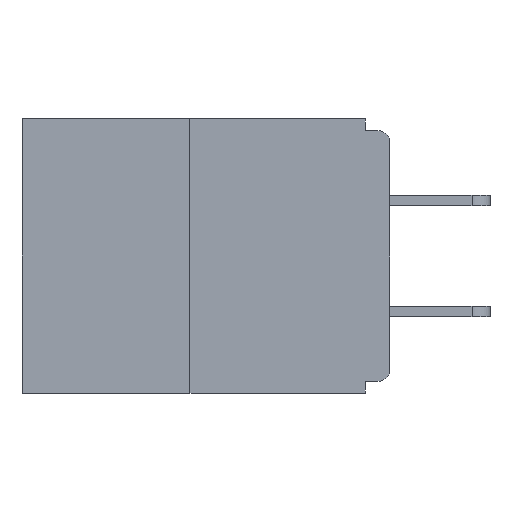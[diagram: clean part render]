
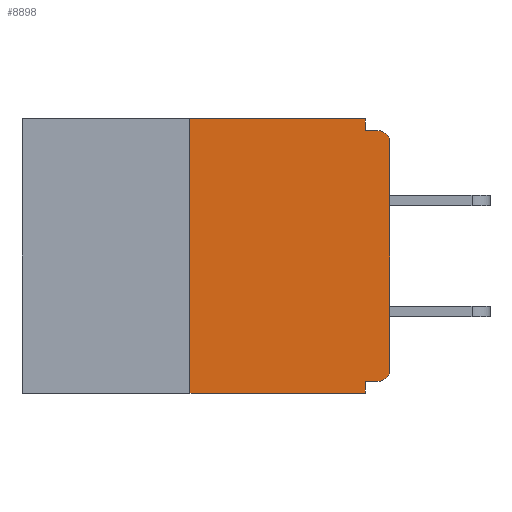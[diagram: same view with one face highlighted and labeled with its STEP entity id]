
A CAD part, left-side view. The second image highlights one B-rep face of the part: STEP entity #8898.
In plain terms, the highlighted planar face has unit normal (-1, 0, 0).
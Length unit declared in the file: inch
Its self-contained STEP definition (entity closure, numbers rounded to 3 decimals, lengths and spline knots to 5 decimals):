
#138 = AXIS2_PLACEMENT_3D ( 'NONE', #9693, #10923, #15683 ) ;
#494 = ORIENTED_EDGE ( 'NONE', *, *, #13513, .T. ) ;
#557 = VERTEX_POINT ( 'NONE', #8828 ) ;
#639 = CARTESIAN_POINT ( 'NONE',  ( 0., 0.46, 0. ) ) ;
#758 = CARTESIAN_POINT ( 'NONE',  ( 0., 0., -0.03 ) ) ;
#788 = VECTOR ( 'NONE', #9981, 39.37008 ) ;
#994 = CARTESIAN_POINT ( 'NONE',  ( 0., 0.25, 0. ) ) ;
#1169 = CARTESIAN_POINT ( 'NONE',  ( 0., 0.015, -0.328 ) ) ;
#1324 = CARTESIAN_POINT ( 'NONE',  ( 0., 0.031, 0. ) ) ;
#1523 = DIRECTION ( 'NONE',  ( 0., -1., 0. ) ) ;
#1751 = VERTEX_POINT ( 'NONE', #758 ) ;
#2694 = LINE ( 'NONE', #13413, #4240 ) ;
#2738 = VERTEX_POINT ( 'NONE', #1169 ) ;
#2758 = EDGE_CURVE ( 'NONE', #14366, #15210, #14642, .T. ) ;
#2929 = DIRECTION ( 'NONE',  ( -1., 0., 0. ) ) ;
#3044 = CARTESIAN_POINT ( 'NONE',  ( 0., 0.25, 0. ) ) ;
#3062 = PLANE ( 'NONE',  #13692 ) ;
#3267 = ORIENTED_EDGE ( 'NONE', *, *, #8157, .F. ) ;
#3478 = DIRECTION ( 'NONE',  ( 0., 0., 1. ) ) ;
#3661 = EDGE_CURVE ( 'NONE', #4261, #11013, #11527, .T. ) ;
#3828 = VERTEX_POINT ( 'NONE', #14357 ) ;
#3891 = ORIENTED_EDGE ( 'NONE', *, *, #13217, .F. ) ;
#4125 = CARTESIAN_POINT ( 'NONE',  ( 0., 0.015, -0.03 ) ) ;
#4240 = VECTOR ( 'NONE', #4927, 39.37008 ) ;
#4261 = VERTEX_POINT ( 'NONE', #12581 ) ;
#4388 = EDGE_CURVE ( 'NONE', #5724, #1751, #14214, .T. ) ;
#4489 = CARTESIAN_POINT ( 'NONE',  ( 0., 0.015, -0.015 ) ) ;
#4735 = FACE_OUTER_BOUND ( 'NONE', #6961, .T. ) ;
#4804 = CIRCLE ( 'NONE', #138, 0.015 ) ;
#4927 = DIRECTION ( 'NONE',  ( 0., 0., -1. ) ) ;
#5104 = ORIENTED_EDGE ( 'NONE', *, *, #3661, .F. ) ;
#5170 = DIRECTION ( 'NONE',  ( 0., -1., 0. ) ) ;
#5554 = ORIENTED_EDGE ( 'NONE', *, *, #11014, .F. ) ;
#5724 = VERTEX_POINT ( 'NONE', #14810 ) ;
#6026 = CARTESIAN_POINT ( 'NONE',  ( 0., 0., -0.015 ) ) ;
#6124 = ORIENTED_EDGE ( 'NONE', *, *, #11642, .F. ) ;
#6230 = ORIENTED_EDGE ( 'NONE', *, *, #12627, .T. ) ;
#6364 = LINE ( 'NONE', #15581, #13522 ) ;
#6420 = ORIENTED_EDGE ( 'NONE', *, *, #4388, .T. ) ;
#6907 = DIRECTION ( 'NONE',  ( 0., 0., -1. ) ) ;
#6934 = LINE ( 'NONE', #1324, #788 ) ;
#6961 = EDGE_LOOP ( 'NONE', ( #3267, #5104, #12795, #3891, #5554, #6230, #6420, #494, #7894, #6124 ) ) ;
#7649 = VECTOR ( 'NONE', #3478, 39.37008 ) ;
#7894 = ORIENTED_EDGE ( 'NONE', *, *, #2758, .F. ) ;
#7984 = CARTESIAN_POINT ( 'NONE',  ( 0., 0., -0.328 ) ) ;
#8157 = EDGE_CURVE ( 'NONE', #11013, #13933, #6364, .T. ) ;
#8723 = EDGE_CURVE ( 'NONE', #4261, #3828, #14931, .T. ) ;
#8828 = CARTESIAN_POINT ( 'NONE',  ( 0., 0.031, -0.328 ) ) ;
#8898 = ADVANCED_FACE ( 'NONE', ( #4735 ), #3062, .F. ) ;
#9211 = CARTESIAN_POINT ( 'NONE',  ( 0., 0., 0. ) ) ;
#9340 = CARTESIAN_POINT ( 'NONE',  ( 0., 0.031, 0. ) ) ;
#9513 = VECTOR ( 'NONE', #5170, 39.37008 ) ;
#9693 = CARTESIAN_POINT ( 'NONE',  ( 0., 0.015, -0.313 ) ) ;
#9981 = DIRECTION ( 'NONE',  ( 0., 0., -1. ) ) ;
#10098 = CARTESIAN_POINT ( 'NONE',  ( 0., 0.46, -0.343 ) ) ;
#10345 = CARTESIAN_POINT ( 'NONE',  ( 0., 0.031, -0.015 ) ) ;
#10605 = DIRECTION ( 'NONE',  ( 1., 0., 0. ) ) ;
#10923 = DIRECTION ( 'NONE',  ( -1., 0., 0. ) ) ;
#10929 = DIRECTION ( 'NONE',  ( 0., -1., 0. ) ) ;
#10933 = VECTOR ( 'NONE', #12848, 39.37008 ) ;
#11013 = VERTEX_POINT ( 'NONE', #3044 ) ;
#11014 = EDGE_CURVE ( 'NONE', #2738, #557, #13173, .T. ) ;
#11351 = VECTOR ( 'NONE', #10929, 39.37008 ) ;
#11504 = AXIS2_PLACEMENT_3D ( 'NONE', #4125, #2929, #12748 ) ;
#11527 = LINE ( 'NONE', #994, #7649 ) ;
#11642 = EDGE_CURVE ( 'NONE', #13933, #14366, #6934, .T. ) ;
#11821 = DIRECTION ( 'NONE',  ( 0., 1., 0. ) ) ;
#12119 = CIRCLE ( 'NONE', #11504, 0.015 ) ;
#12581 = CARTESIAN_POINT ( 'NONE',  ( 0., 0.25, -0.343 ) ) ;
#12627 = EDGE_CURVE ( 'NONE', #2738, #5724, #4804, .T. ) ;
#12748 = DIRECTION ( 'NONE',  ( 0., 0., -1. ) ) ;
#12795 = ORIENTED_EDGE ( 'NONE', *, *, #8723, .T. ) ;
#12848 = DIRECTION ( 'NONE',  ( 0., 0., 1. ) ) ;
#13173 = LINE ( 'NONE', #7984, #14326 ) ;
#13217 = EDGE_CURVE ( 'NONE', #557, #3828, #2694, .T. ) ;
#13413 = CARTESIAN_POINT ( 'NONE',  ( 0., 0.031, -0.343 ) ) ;
#13513 = EDGE_CURVE ( 'NONE', #1751, #15210, #12119, .T. ) ;
#13522 = VECTOR ( 'NONE', #1523, 39.37008 ) ;
#13692 = AXIS2_PLACEMENT_3D ( 'NONE', #639, #10605, #6907 ) ;
#13933 = VERTEX_POINT ( 'NONE', #9340 ) ;
#14214 = LINE ( 'NONE', #9211, #10933 ) ;
#14326 = VECTOR ( 'NONE', #11821, 39.37008 ) ;
#14357 = CARTESIAN_POINT ( 'NONE',  ( 0., 0.031, -0.343 ) ) ;
#14366 = VERTEX_POINT ( 'NONE', #10345 ) ;
#14642 = LINE ( 'NONE', #6026, #11351 ) ;
#14810 = CARTESIAN_POINT ( 'NONE',  ( 0., 0., -0.313 ) ) ;
#14931 = LINE ( 'NONE', #10098, #9513 ) ;
#15210 = VERTEX_POINT ( 'NONE', #4489 ) ;
#15581 = CARTESIAN_POINT ( 'NONE',  ( 0., 0.46, 0. ) ) ;
#15683 = DIRECTION ( 'NONE',  ( 0., 0., -1. ) ) ;
